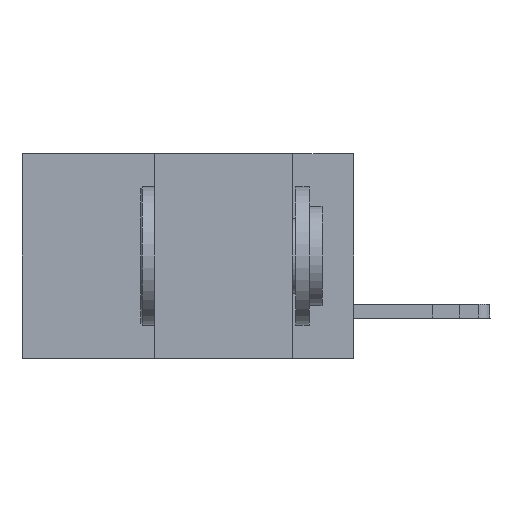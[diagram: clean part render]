
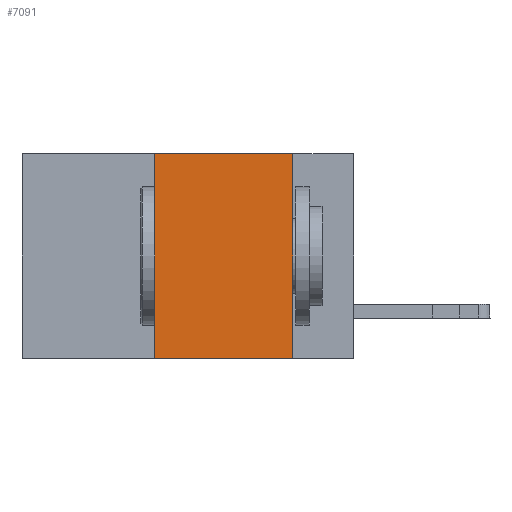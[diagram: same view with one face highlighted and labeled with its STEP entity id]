
A CAD part, left-side view. The second image highlights one B-rep face of the part: STEP entity #7091.
In plain terms, the highlighted planar face has unit normal (-1, 0, 0).
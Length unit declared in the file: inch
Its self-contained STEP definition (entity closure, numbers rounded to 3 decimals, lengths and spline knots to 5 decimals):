
#509 = EDGE_LOOP ( 'NONE', ( #2504, #14392, #5780, #5284 ) ) ;
#705 = CARTESIAN_POINT ( 'NONE',  ( 0., 0.11, 0. ) ) ;
#1282 = CARTESIAN_POINT ( 'NONE',  ( 0., 0.36, 0. ) ) ;
#2504 = ORIENTED_EDGE ( 'NONE', *, *, #12408, .F. ) ;
#2853 = DIRECTION ( 'NONE',  ( 0., 0., 1. ) ) ;
#3197 = VECTOR ( 'NONE', #10935, 39.37008 ) ;
#3201 = VERTEX_POINT ( 'NONE', #11903 ) ;
#3812 = CARTESIAN_POINT ( 'NONE',  ( 0., 0.36, 0. ) ) ;
#4216 = LINE ( 'NONE', #15444, #3197 ) ;
#4438 = VERTEX_POINT ( 'NONE', #3812 ) ;
#5284 = ORIENTED_EDGE ( 'NONE', *, *, #14192, .T. ) ;
#5780 = ORIENTED_EDGE ( 'NONE', *, *, #12791, .F. ) ;
#6750 = VECTOR ( 'NONE', #2853, 39.37008 ) ;
#6795 = AXIS2_PLACEMENT_3D ( 'NONE', #19075, #16120, #7044 ) ;
#7044 = DIRECTION ( 'NONE',  ( 0., 0., -1. ) ) ;
#7051 = VECTOR ( 'NONE', #12501, 39.37008 ) ;
#7091 = ADVANCED_FACE ( 'NONE', ( #18596 ), #13063, .F. ) ;
#7466 = EDGE_CURVE ( 'NONE', #4438, #19698, #4216, .T. ) ;
#9373 = LINE ( 'NONE', #18611, #13415 ) ;
#9527 = DIRECTION ( 'NONE',  ( 0., 0., -1. ) ) ;
#10935 = DIRECTION ( 'NONE',  ( 0., -1., 0. ) ) ;
#10996 = CARTESIAN_POINT ( 'NONE',  ( 0., 0.6, -0.37 ) ) ;
#11903 = CARTESIAN_POINT ( 'NONE',  ( 0., 0.36, -0.37 ) ) ;
#12408 = EDGE_CURVE ( 'NONE', #19698, #15452, #9373, .T. ) ;
#12501 = DIRECTION ( 'NONE',  ( 0., -1., 0. ) ) ;
#12791 = EDGE_CURVE ( 'NONE', #3201, #4438, #18837, .T. ) ;
#13063 = PLANE ( 'NONE',  #6795 ) ;
#13415 = VECTOR ( 'NONE', #9527, 39.37008 ) ;
#14192 = EDGE_CURVE ( 'NONE', #3201, #15452, #18657, .T. ) ;
#14392 = ORIENTED_EDGE ( 'NONE', *, *, #7466, .F. ) ;
#15444 = CARTESIAN_POINT ( 'NONE',  ( 0., 0.6, 0. ) ) ;
#15452 = VERTEX_POINT ( 'NONE', #15646 ) ;
#15646 = CARTESIAN_POINT ( 'NONE',  ( 0., 0.11, -0.37 ) ) ;
#16120 = DIRECTION ( 'NONE',  ( 1., 0., 0. ) ) ;
#18596 = FACE_OUTER_BOUND ( 'NONE', #509, .T. ) ;
#18611 = CARTESIAN_POINT ( 'NONE',  ( 0., 0.11, 0. ) ) ;
#18657 = LINE ( 'NONE', #10996, #7051 ) ;
#18837 = LINE ( 'NONE', #1282, #6750 ) ;
#19075 = CARTESIAN_POINT ( 'NONE',  ( 0., 0.6, 0. ) ) ;
#19698 = VERTEX_POINT ( 'NONE', #705 ) ;
